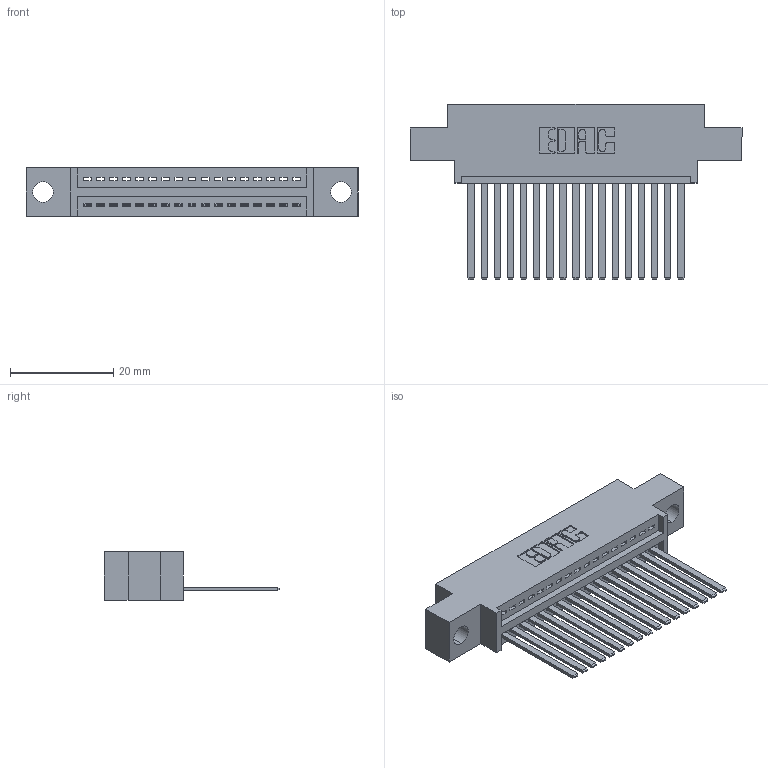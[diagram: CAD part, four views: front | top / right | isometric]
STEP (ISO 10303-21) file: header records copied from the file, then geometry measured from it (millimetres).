
FILE_DESCRIPTION (( 'STEP AP203' ), '1' );
FILE_NAME ('345-017-544-604.STEP', '2018-08-19T04:22:30', ( '' ), ( '' ), 'SwSTEP 2.0', 'SolidWorks 2016', '' );
FILE_SCHEMA (( 'CONFIG_CONTROL_DESIGN' ));
Length unit declared in the file: inch
Products named in the file (3): 345 Part_0.170 Offset - 0.156 Dia-TH; 345-292-001_345-293-144; 345-017-544-604
Assembly tree (18 placements, depth 2):
  345-017-544-604
    345 Part_0.170 Offset - 0.156 Dia-TH
    345-292-001_345-293-144  x17
Bounding box: 64.39 x 33.96 x 9.4 mm (x, y, z)
Volume: 5906.6 mm3; surface area: 8035.9 mm2
Topology: 18 solids, 18 shells, 1014 faces, 3039 edges, 2002 vertices
Faces by surface type: plane 696, cylinder 318
Entity records: 16111 total; most frequent: CARTESIAN_POINT 2799, ORIENTED_EDGE 2750, DIRECTION 2477, EDGE_CURVE 1375, VECTOR 1179, LINE 1179, VERTEX_POINT 914, AXIS2_PLACEMENT_3D 649
